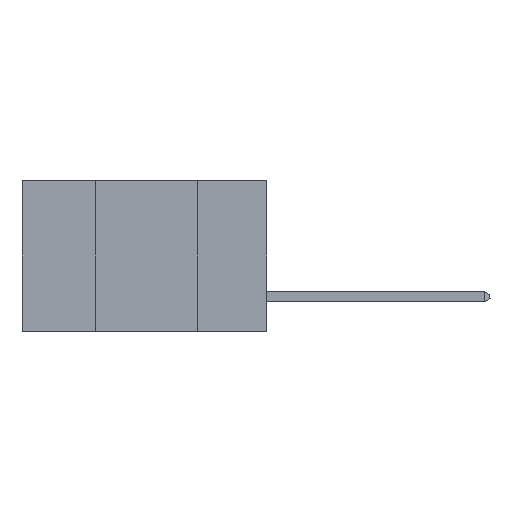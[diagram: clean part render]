
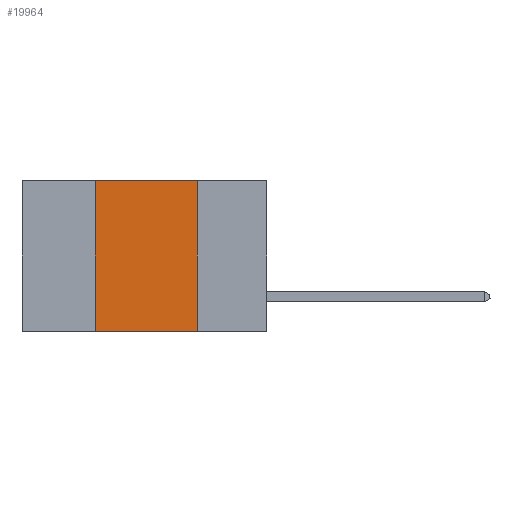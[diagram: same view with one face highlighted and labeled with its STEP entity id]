
A CAD part, left-side view. The second image highlights one B-rep face of the part: STEP entity #19964.
In plain terms, the highlighted planar face has unit normal (-1, 0, 0).
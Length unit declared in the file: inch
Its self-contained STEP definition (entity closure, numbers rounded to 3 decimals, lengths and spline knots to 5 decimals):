
#495 = DIRECTION ( 'NONE',  ( 0., -1., 0. ) ) ;
#660 = CARTESIAN_POINT ( 'NONE',  ( 0., 0.6, 0. ) ) ;
#1812 = CARTESIAN_POINT ( 'NONE',  ( 0., 0.6, 0. ) ) ;
#2649 = EDGE_LOOP ( 'NONE', ( #21444, #20489, #17737, #5488 ) ) ;
#3424 = LINE ( 'NONE', #4894, #13718 ) ;
#4539 = VERTEX_POINT ( 'NONE', #6078 ) ;
#4894 = CARTESIAN_POINT ( 'NONE',  ( 0., 0.17, 0. ) ) ;
#5488 = ORIENTED_EDGE ( 'NONE', *, *, #15169, .T. ) ;
#5864 = EDGE_CURVE ( 'NONE', #18592, #5922, #15903, .T. ) ;
#5922 = VERTEX_POINT ( 'NONE', #6100 ) ;
#6078 = CARTESIAN_POINT ( 'NONE',  ( 0., 0.17, -0.37 ) ) ;
#6100 = CARTESIAN_POINT ( 'NONE',  ( 0., 0.42, 0. ) ) ;
#6548 = EDGE_CURVE ( 'NONE', #21884, #4539, #3424, .T. ) ;
#7158 = DIRECTION ( 'NONE',  ( 0., -1., 0. ) ) ;
#8175 = DIRECTION ( 'NONE',  ( 0., 0., -1. ) ) ;
#8714 = LINE ( 'NONE', #660, #13856 ) ;
#8720 = DIRECTION ( 'NONE',  ( 1., 0., 0. ) ) ;
#9353 = CARTESIAN_POINT ( 'NONE',  ( 0., 0.42, 0. ) ) ;
#9699 = CARTESIAN_POINT ( 'NONE',  ( 0., 0.42, -0.37 ) ) ;
#10483 = AXIS2_PLACEMENT_3D ( 'NONE', #1812, #8720, #15664 ) ;
#12622 = DIRECTION ( 'NONE',  ( 0., 0., 1. ) ) ;
#13712 = PLANE ( 'NONE',  #10483 ) ;
#13718 = VECTOR ( 'NONE', #8175, 39.37008 ) ;
#13856 = VECTOR ( 'NONE', #495, 39.37008 ) ;
#15111 = VECTOR ( 'NONE', #12622, 39.37008 ) ;
#15169 = EDGE_CURVE ( 'NONE', #18592, #4539, #18980, .T. ) ;
#15664 = DIRECTION ( 'NONE',  ( 0., 0., -1. ) ) ;
#15903 = LINE ( 'NONE', #9353, #15111 ) ;
#15915 = CARTESIAN_POINT ( 'NONE',  ( 0., 0.17, 0. ) ) ;
#17323 = FACE_OUTER_BOUND ( 'NONE', #2649, .T. ) ;
#17737 = ORIENTED_EDGE ( 'NONE', *, *, #5864, .F. ) ;
#18449 = VECTOR ( 'NONE', #7158, 39.37008 ) ;
#18592 = VERTEX_POINT ( 'NONE', #9699 ) ;
#18980 = LINE ( 'NONE', #22205, #18449 ) ;
#19042 = EDGE_CURVE ( 'NONE', #5922, #21884, #8714, .T. ) ;
#19964 = ADVANCED_FACE ( 'NONE', ( #17323 ), #13712, .F. ) ;
#20489 = ORIENTED_EDGE ( 'NONE', *, *, #19042, .F. ) ;
#21444 = ORIENTED_EDGE ( 'NONE', *, *, #6548, .F. ) ;
#21884 = VERTEX_POINT ( 'NONE', #15915 ) ;
#22205 = CARTESIAN_POINT ( 'NONE',  ( 0., 0.6, -0.37 ) ) ;
